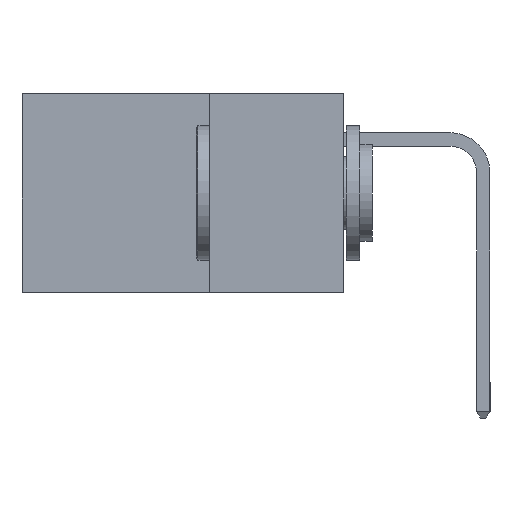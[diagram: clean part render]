
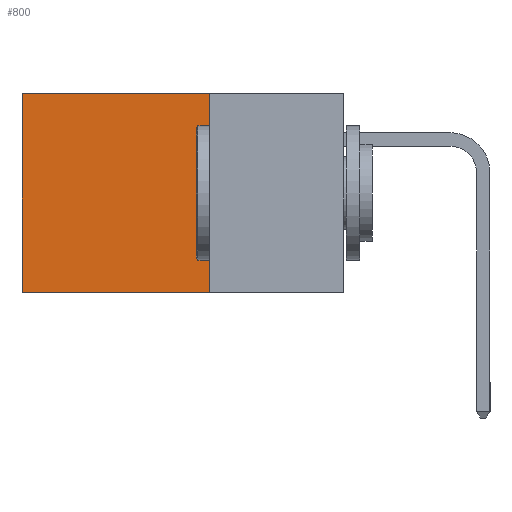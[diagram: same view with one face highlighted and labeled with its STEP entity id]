
A CAD part, left-side view. The second image highlights one B-rep face of the part: STEP entity #800.
In plain terms, the highlighted planar face has unit normal (-1, 0, 0).
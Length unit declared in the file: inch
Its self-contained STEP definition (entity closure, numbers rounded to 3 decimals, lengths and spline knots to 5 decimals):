
#584 = EDGE_CURVE ( 'NONE', #10894, #5651, #11367, .T. ) ;
#636 = ORIENTED_EDGE ( 'NONE', *, *, #3323, .T. ) ;
#800 = ADVANCED_FACE ( 'NONE', ( #11994 ), #11494, .F. ) ;
#962 = DIRECTION ( 'NONE',  ( 0., 0., -1. ) ) ;
#1154 = ORIENTED_EDGE ( 'NONE', *, *, #584, .T. ) ;
#2447 = ORIENTED_EDGE ( 'NONE', *, *, #14563, .F. ) ;
#2701 = VERTEX_POINT ( 'NONE', #11173 ) ;
#3323 = EDGE_CURVE ( 'NONE', #10331, #10894, #8593, .T. ) ;
#3446 = LINE ( 'NONE', #5008, #14345 ) ;
#3644 = DIRECTION ( 'NONE',  ( 0., 0., -1. ) ) ;
#3848 = VECTOR ( 'NONE', #12548, 39.37008 ) ;
#5008 = CARTESIAN_POINT ( 'NONE',  ( 0.298, 0.25, -0.37 ) ) ;
#5651 = VERTEX_POINT ( 'NONE', #9063 ) ;
#6467 = DIRECTION ( 'NONE',  ( 0., 1., 0. ) ) ;
#8099 = CARTESIAN_POINT ( 'NONE',  ( 0.298, 0.25, 0. ) ) ;
#8593 = LINE ( 'NONE', #18394, #3848 ) ;
#8612 = EDGE_CURVE ( 'NONE', #10331, #2701, #16161, .T. ) ;
#9021 = AXIS2_PLACEMENT_3D ( 'NONE', #10649, #13512, #13465 ) ;
#9063 = CARTESIAN_POINT ( 'NONE',  ( 0.298, 0.6, -0.37 ) ) ;
#10331 = VERTEX_POINT ( 'NONE', #17921 ) ;
#10649 = CARTESIAN_POINT ( 'NONE',  ( 0.298, 0.25, 0. ) ) ;
#10706 = CARTESIAN_POINT ( 'NONE',  ( 0.298, 0.6, 0. ) ) ;
#10894 = VERTEX_POINT ( 'NONE', #10706 ) ;
#11173 = CARTESIAN_POINT ( 'NONE',  ( 0.298, 0.25, -0.37 ) ) ;
#11367 = LINE ( 'NONE', #14543, #18388 ) ;
#11494 = PLANE ( 'NONE',  #9021 ) ;
#11994 = FACE_OUTER_BOUND ( 'NONE', #17696, .T. ) ;
#12006 = VECTOR ( 'NONE', #962, 39.37008 ) ;
#12548 = DIRECTION ( 'NONE',  ( 0., 1., 0. ) ) ;
#13465 = DIRECTION ( 'NONE',  ( 0., 0., -1. ) ) ;
#13512 = DIRECTION ( 'NONE',  ( 1., 0., 0. ) ) ;
#14345 = VECTOR ( 'NONE', #6467, 39.37008 ) ;
#14467 = ORIENTED_EDGE ( 'NONE', *, *, #8612, .F. ) ;
#14543 = CARTESIAN_POINT ( 'NONE',  ( 0.298, 0.6, 0. ) ) ;
#14563 = EDGE_CURVE ( 'NONE', #2701, #5651, #3446, .T. ) ;
#16161 = LINE ( 'NONE', #8099, #12006 ) ;
#17696 = EDGE_LOOP ( 'NONE', ( #1154, #2447, #14467, #636 ) ) ;
#17921 = CARTESIAN_POINT ( 'NONE',  ( 0.298, 0.25, 0. ) ) ;
#18388 = VECTOR ( 'NONE', #3644, 39.37008 ) ;
#18394 = CARTESIAN_POINT ( 'NONE',  ( 0.298, 0.25, 0. ) ) ;
